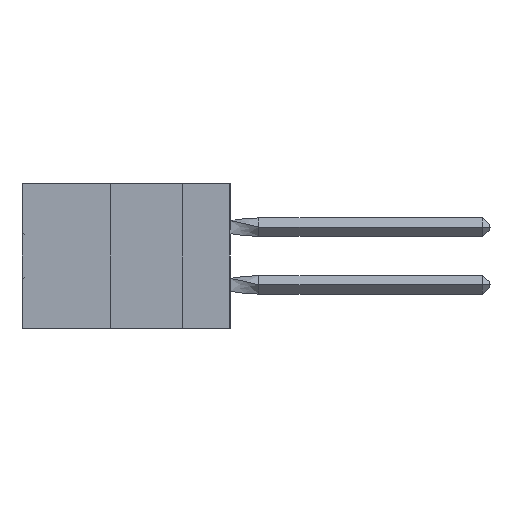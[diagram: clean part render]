
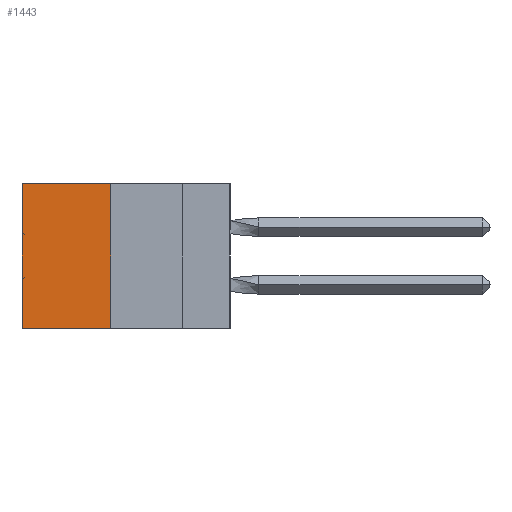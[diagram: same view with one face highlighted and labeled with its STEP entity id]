
A CAD part, left-side view. The second image highlights one B-rep face of the part: STEP entity #1443.
In plain terms, the highlighted planar face has unit normal (-1, 0, 0).
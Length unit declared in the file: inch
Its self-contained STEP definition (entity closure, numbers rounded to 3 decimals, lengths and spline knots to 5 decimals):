
#1443 = ADVANCED_FACE ( 'NONE', ( #49948 ), #35220, .F. ) ;
#2932 = EDGE_CURVE ( 'NONE', #47458, #32210, #27166, .T. ) ;
#4052 = CARTESIAN_POINT ( 'NONE',  ( 0.305, 0.72, 0. ) ) ;
#4678 = DIRECTION ( 'NONE',  ( 1., 0., 0. ) ) ;
#7040 = VECTOR ( 'NONE', #17397, 39.37008 ) ;
#7068 = EDGE_LOOP ( 'NONE', ( #26876, #43607, #36483, #45750 ) ) ;
#7426 = DIRECTION ( 'NONE',  ( 0., 0., -1. ) ) ;
#11051 = LINE ( 'NONE', #50559, #7040 ) ;
#11080 = VERTEX_POINT ( 'NONE', #47979 ) ;
#12758 = LINE ( 'NONE', #41230, #26932 ) ;
#12776 = CARTESIAN_POINT ( 'NONE',  ( 0.305, 0.72, -0.5 ) ) ;
#15385 = CARTESIAN_POINT ( 'NONE',  ( 0.305, 0.413, -0.5 ) ) ;
#16824 = EDGE_CURVE ( 'NONE', #11080, #47458, #11051, .T. ) ;
#17107 = DIRECTION ( 'NONE',  ( 0., 0., -1. ) ) ;
#17397 = DIRECTION ( 'NONE',  ( 0., 1., 0. ) ) ;
#23630 = VERTEX_POINT ( 'NONE', #15385 ) ;
#25073 = CARTESIAN_POINT ( 'NONE',  ( 0.305, 0.413, -0.5 ) ) ;
#26872 = CARTESIAN_POINT ( 'NONE',  ( 0.305, 0.72, -0.5 ) ) ;
#26876 = ORIENTED_EDGE ( 'NONE', *, *, #2932, .T. ) ;
#26932 = VECTOR ( 'NONE', #53931, 39.37008 ) ;
#27166 = LINE ( 'NONE', #12776, #34485 ) ;
#30401 = EDGE_CURVE ( 'NONE', #11080, #23630, #38578, .T. ) ;
#30747 = DIRECTION ( 'NONE',  ( 0., 0., -1. ) ) ;
#32024 = AXIS2_PLACEMENT_3D ( 'NONE', #39520, #4678, #30747 ) ;
#32210 = VERTEX_POINT ( 'NONE', #26872 ) ;
#34485 = VECTOR ( 'NONE', #17107, 39.37008 ) ;
#34532 = VECTOR ( 'NONE', #7426, 39.37008 ) ;
#35220 = PLANE ( 'NONE',  #32024 ) ;
#36483 = ORIENTED_EDGE ( 'NONE', *, *, #30401, .F. ) ;
#38578 = LINE ( 'NONE', #25073, #34532 ) ;
#39520 = CARTESIAN_POINT ( 'NONE',  ( 0.305, 0.413, -0.5 ) ) ;
#41230 = CARTESIAN_POINT ( 'NONE',  ( 0.305, 0.413, -0.5 ) ) ;
#43607 = ORIENTED_EDGE ( 'NONE', *, *, #55202, .F. ) ;
#45750 = ORIENTED_EDGE ( 'NONE', *, *, #16824, .T. ) ;
#47458 = VERTEX_POINT ( 'NONE', #4052 ) ;
#47979 = CARTESIAN_POINT ( 'NONE',  ( 0.305, 0.413, 0. ) ) ;
#49948 = FACE_OUTER_BOUND ( 'NONE', #7068, .T. ) ;
#50559 = CARTESIAN_POINT ( 'NONE',  ( 0.305, 0.413, 0. ) ) ;
#53931 = DIRECTION ( 'NONE',  ( 0., 1., 0. ) ) ;
#55202 = EDGE_CURVE ( 'NONE', #23630, #32210, #12758, .T. ) ;
